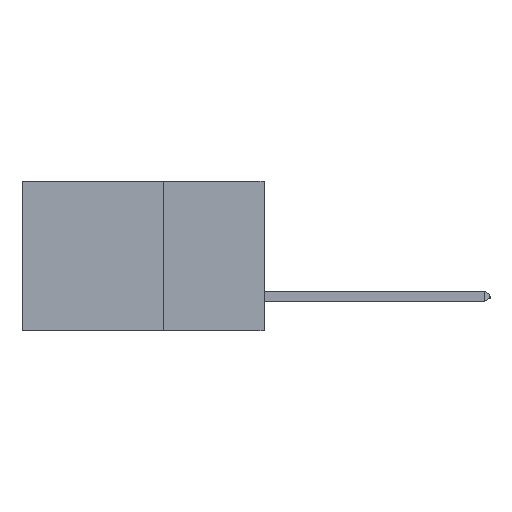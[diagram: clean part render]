
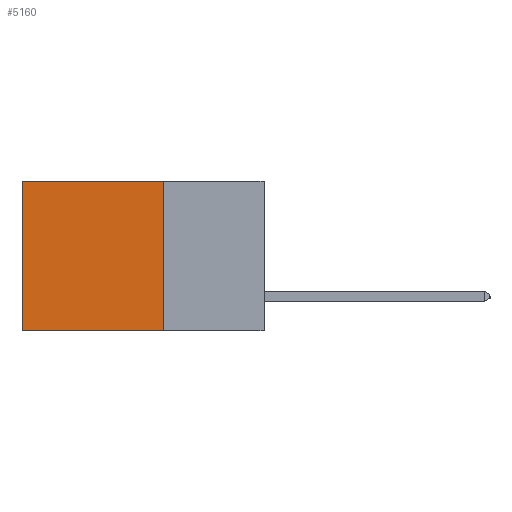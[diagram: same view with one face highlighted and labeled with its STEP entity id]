
A CAD part, left-side view. The second image highlights one B-rep face of the part: STEP entity #5160.
In plain terms, the highlighted planar face has unit normal (-1, 0, 0).
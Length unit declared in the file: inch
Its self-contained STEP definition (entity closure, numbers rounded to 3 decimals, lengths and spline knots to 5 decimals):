
#888 = CARTESIAN_POINT ( 'NONE',  ( 0.298, 0.6, 0. ) ) ;
#1282 = DIRECTION ( 'NONE',  ( 0., 0., -1. ) ) ;
#1360 = EDGE_CURVE ( 'NONE', #11162, #9780, #8007, .T. ) ;
#1513 = DIRECTION ( 'NONE',  ( 1., 0., 0. ) ) ;
#2529 = CARTESIAN_POINT ( 'NONE',  ( 0.298, 0.25, 0. ) ) ;
#4281 = EDGE_LOOP ( 'NONE', ( #9884, #20389, #13798, #20186 ) ) ;
#4964 = DIRECTION ( 'NONE',  ( 0., 1., 0. ) ) ;
#5060 = DIRECTION ( 'NONE',  ( 0., 0., -1. ) ) ;
#5160 = ADVANCED_FACE ( 'NONE', ( #16557 ), #11872, .F. ) ;
#8007 = LINE ( 'NONE', #888, #21336 ) ;
#8884 = VECTOR ( 'NONE', #5060, 39.37008 ) ;
#9424 = LINE ( 'NONE', #18605, #8884 ) ;
#9780 = VERTEX_POINT ( 'NONE', #10225 ) ;
#9884 = ORIENTED_EDGE ( 'NONE', *, *, #1360, .T. ) ;
#10060 = CARTESIAN_POINT ( 'NONE',  ( 0.298, 0.25, -0.37 ) ) ;
#10225 = CARTESIAN_POINT ( 'NONE',  ( 0.298, 0.6, -0.37 ) ) ;
#10972 = EDGE_CURVE ( 'NONE', #12213, #9780, #18604, .T. ) ;
#11162 = VERTEX_POINT ( 'NONE', #12336 ) ;
#11872 = PLANE ( 'NONE',  #13498 ) ;
#12213 = VERTEX_POINT ( 'NONE', #15468 ) ;
#12336 = CARTESIAN_POINT ( 'NONE',  ( 0.298, 0.6, 0. ) ) ;
#12908 = DIRECTION ( 'NONE',  ( 0., 1., 0. ) ) ;
#13498 = AXIS2_PLACEMENT_3D ( 'NONE', #18516, #1513, #13613 ) ;
#13613 = DIRECTION ( 'NONE',  ( 0., 0., -1. ) ) ;
#13798 = ORIENTED_EDGE ( 'NONE', *, *, #17326, .F. ) ;
#14237 = VECTOR ( 'NONE', #4964, 39.37008 ) ;
#15168 = CARTESIAN_POINT ( 'NONE',  ( 0.298, 0.25, 0. ) ) ;
#15468 = CARTESIAN_POINT ( 'NONE',  ( 0.298, 0.25, -0.37 ) ) ;
#15831 = LINE ( 'NONE', #2529, #18627 ) ;
#16557 = FACE_OUTER_BOUND ( 'NONE', #4281, .T. ) ;
#17055 = EDGE_CURVE ( 'NONE', #19709, #11162, #15831, .T. ) ;
#17326 = EDGE_CURVE ( 'NONE', #19709, #12213, #9424, .T. ) ;
#18516 = CARTESIAN_POINT ( 'NONE',  ( 0.298, 0.25, 0. ) ) ;
#18604 = LINE ( 'NONE', #10060, #14237 ) ;
#18605 = CARTESIAN_POINT ( 'NONE',  ( 0.298, 0.25, 0. ) ) ;
#18627 = VECTOR ( 'NONE', #12908, 39.37008 ) ;
#19709 = VERTEX_POINT ( 'NONE', #15168 ) ;
#20186 = ORIENTED_EDGE ( 'NONE', *, *, #17055, .T. ) ;
#20389 = ORIENTED_EDGE ( 'NONE', *, *, #10972, .F. ) ;
#21336 = VECTOR ( 'NONE', #1282, 39.37008 ) ;
